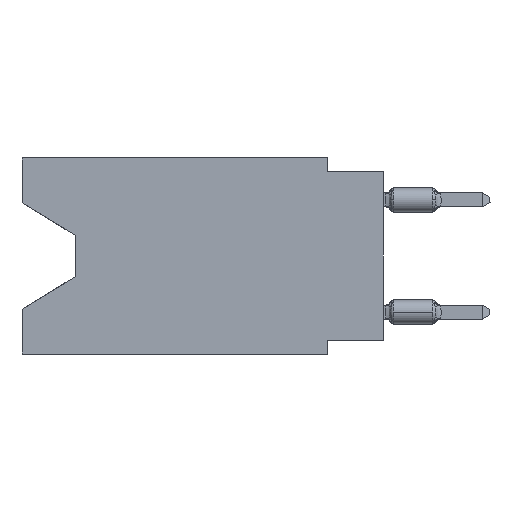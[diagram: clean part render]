
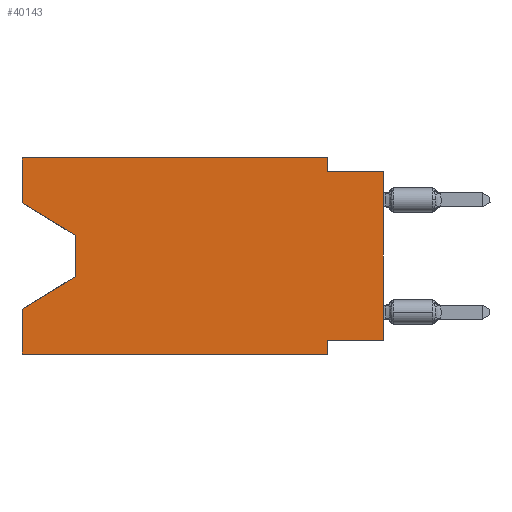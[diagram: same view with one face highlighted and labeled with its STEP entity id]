
A CAD part, left-side view. The second image highlights one B-rep face of the part: STEP entity #40143.
In plain terms, the highlighted planar face has unit normal (-1, 0, 0).
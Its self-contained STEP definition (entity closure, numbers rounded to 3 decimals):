
#113 = LINE ( 'NONE', #17039, #24678 ) ;
#588 = VERTEX_POINT ( 'NONE', #21056 ) ;
#630 = EDGE_CURVE ( 'NONE', #1290, #9018, #39254, .T. ) ;
#1038 = ORIENTED_EDGE ( 'NONE', *, *, #38472, .T. ) ;
#1092 = DIRECTION ( 'NONE',  ( 0., 0., 1. ) ) ;
#1290 = VERTEX_POINT ( 'NONE', #27605 ) ;
#1809 = VECTOR ( 'NONE', #13258, 1000. ) ;
#1930 = ORIENTED_EDGE ( 'NONE', *, *, #27850, .T. ) ;
#2614 = ORIENTED_EDGE ( 'NONE', *, *, #630, .F. ) ;
#5029 = PLANE ( 'NONE',  #36542 ) ;
#5314 = VECTOR ( 'NONE', #26515, 1000. ) ;
#5423 = VERTEX_POINT ( 'NONE', #18499 ) ;
#5823 = LINE ( 'NONE', #12523, #5314 ) ;
#5864 = LINE ( 'NONE', #8759, #38776 ) ;
#7186 = EDGE_CURVE ( 'NONE', #26577, #5423, #24933, .T. ) ;
#7244 = CARTESIAN_POINT ( 'NONE',  ( 0., 16.383, 0. ) ) ;
#7742 = CARTESIAN_POINT ( 'NONE',  ( 0., 0., -8.255 ) ) ;
#8458 = VECTOR ( 'NONE', #39185, 1000. ) ;
#8560 = DIRECTION ( 'NONE',  ( 0., 0., -1. ) ) ;
#8759 = CARTESIAN_POINT ( 'NONE',  ( 0., 13.97, -5.385 ) ) ;
#8957 = EDGE_CURVE ( 'NONE', #38007, #27859, #5823, .T. ) ;
#9018 = VERTEX_POINT ( 'NONE', #19012 ) ;
#9893 = VECTOR ( 'NONE', #8560, 1000. ) ;
#10356 = EDGE_CURVE ( 'NONE', #5423, #12263, #5864, .T. ) ;
#10676 = VERTEX_POINT ( 'NONE', #42977 ) ;
#11389 = LINE ( 'NONE', #31603, #1809 ) ;
#12263 = VERTEX_POINT ( 'NONE', #33851 ) ;
#12523 = CARTESIAN_POINT ( 'NONE',  ( 0., 0., -0.635 ) ) ;
#12874 = CARTESIAN_POINT ( 'NONE',  ( 0., 16.383, 0. ) ) ;
#13258 = DIRECTION ( 'NONE',  ( 0., 0., 1. ) ) ;
#13326 = EDGE_CURVE ( 'NONE', #35288, #12263, #11389, .T. ) ;
#13667 = CARTESIAN_POINT ( 'NONE',  ( 0., 13.97, -3.505 ) ) ;
#14583 = VERTEX_POINT ( 'NONE', #33932 ) ;
#15830 = CARTESIAN_POINT ( 'NONE',  ( 0., 2.54, 0. ) ) ;
#16354 = VERTEX_POINT ( 'NONE', #7742 ) ;
#16783 = VECTOR ( 'NONE', #21916, 1000. ) ;
#17039 = CARTESIAN_POINT ( 'NONE',  ( 0., 16.383, -8.89 ) ) ;
#17949 = ORIENTED_EDGE ( 'NONE', *, *, #13326, .F. ) ;
#18113 = VECTOR ( 'NONE', #25569, 1000. ) ;
#18206 = VECTOR ( 'NONE', #1092, 1000. ) ;
#18499 = CARTESIAN_POINT ( 'NONE',  ( 0., 13.97, -5.385 ) ) ;
#18603 = CARTESIAN_POINT ( 'NONE',  ( 0., 16.383, 0. ) ) ;
#18662 = CARTESIAN_POINT ( 'NONE',  ( 0., 0., 0. ) ) ;
#18694 = CARTESIAN_POINT ( 'NONE',  ( 0., 13.97, -3.505 ) ) ;
#18727 = LINE ( 'NONE', #15830, #8458 ) ;
#18799 = CARTESIAN_POINT ( 'NONE',  ( 0., 2.54, -8.89 ) ) ;
#19012 = CARTESIAN_POINT ( 'NONE',  ( 0., 2.54, -8.89 ) ) ;
#20258 = EDGE_CURVE ( 'NONE', #14583, #588, #43354, .T. ) ;
#20448 = CARTESIAN_POINT ( 'NONE',  ( 0., 0., -0.635 ) ) ;
#20654 = VECTOR ( 'NONE', #26421, 1000. ) ;
#20828 = DIRECTION ( 'NONE',  ( 0., 0., 1. ) ) ;
#21056 = CARTESIAN_POINT ( 'NONE',  ( 0., 2.54, 0. ) ) ;
#21603 = EDGE_CURVE ( 'NONE', #10676, #14583, #27075, .T. ) ;
#21916 = DIRECTION ( 'NONE',  ( 0., -0.855, -0.519 ) ) ;
#21948 = FACE_OUTER_BOUND ( 'NONE', #24569, .T. ) ;
#22223 = LINE ( 'NONE', #42487, #18113 ) ;
#23907 = DIRECTION ( 'NONE',  ( 0., -1., 0. ) ) ;
#23985 = DIRECTION ( 'NONE',  ( 0., 0., -1. ) ) ;
#24569 = EDGE_LOOP ( 'NONE', ( #1930, #37198, #30678, #17949, #1038, #2614, #41704, #26914, #26641, #42467, #36585, #42893 ) ) ;
#24678 = VECTOR ( 'NONE', #23907, 1000. ) ;
#24933 = LINE ( 'NONE', #18694, #37962 ) ;
#25569 = DIRECTION ( 'NONE',  ( 0., 1., 0. ) ) ;
#26421 = DIRECTION ( 'NONE',  ( 0., -1., 0. ) ) ;
#26515 = DIRECTION ( 'NONE',  ( 0., -1., 0. ) ) ;
#26577 = VERTEX_POINT ( 'NONE', #13667 ) ;
#26641 = ORIENTED_EDGE ( 'NONE', *, *, #8957, .F. ) ;
#26914 = ORIENTED_EDGE ( 'NONE', *, *, #28625, .T. ) ;
#27075 = LINE ( 'NONE', #7244, #40613 ) ;
#27605 = CARTESIAN_POINT ( 'NONE',  ( 0., 2.54, -8.255 ) ) ;
#27850 = EDGE_CURVE ( 'NONE', #10676, #26577, #34002, .T. ) ;
#27859 = VERTEX_POINT ( 'NONE', #20448 ) ;
#28585 = CARTESIAN_POINT ( 'NONE',  ( 0., 2.54, -0.635 ) ) ;
#28625 = EDGE_CURVE ( 'NONE', #16354, #27859, #28896, .T. ) ;
#28896 = LINE ( 'NONE', #18662, #18206 ) ;
#29688 = DIRECTION ( 'NONE',  ( 0., 0.855, -0.519 ) ) ;
#30678 = ORIENTED_EDGE ( 'NONE', *, *, #10356, .T. ) ;
#31603 = CARTESIAN_POINT ( 'NONE',  ( 0., 16.383, 0. ) ) ;
#32148 = DIRECTION ( 'NONE',  ( 1., 0., 0. ) ) ;
#33851 = CARTESIAN_POINT ( 'NONE',  ( 0., 16.383, -6.852 ) ) ;
#33932 = CARTESIAN_POINT ( 'NONE',  ( 0., 16.383, 0. ) ) ;
#34002 = LINE ( 'NONE', #42380, #16783 ) ;
#34415 = EDGE_CURVE ( 'NONE', #588, #38007, #18727, .T. ) ;
#34551 = CARTESIAN_POINT ( 'NONE',  ( 0., 16.383, -8.89 ) ) ;
#35288 = VERTEX_POINT ( 'NONE', #34551 ) ;
#36542 = AXIS2_PLACEMENT_3D ( 'NONE', #18603, #32148, #23985 ) ;
#36585 = ORIENTED_EDGE ( 'NONE', *, *, #20258, .F. ) ;
#37198 = ORIENTED_EDGE ( 'NONE', *, *, #7186, .T. ) ;
#37962 = VECTOR ( 'NONE', #42510, 1000. ) ;
#38007 = VERTEX_POINT ( 'NONE', #28585 ) ;
#38472 = EDGE_CURVE ( 'NONE', #35288, #9018, #113, .T. ) ;
#38776 = VECTOR ( 'NONE', #29688, 1000. ) ;
#39185 = DIRECTION ( 'NONE',  ( 0., 0., -1. ) ) ;
#39254 = LINE ( 'NONE', #18799, #9893 ) ;
#40143 = ADVANCED_FACE ( 'NONE', ( #21948 ), #5029, .F. ) ;
#40613 = VECTOR ( 'NONE', #20828, 1000. ) ;
#41704 = ORIENTED_EDGE ( 'NONE', *, *, #42107, .F. ) ;
#42107 = EDGE_CURVE ( 'NONE', #16354, #1290, #22223, .T. ) ;
#42380 = CARTESIAN_POINT ( 'NONE',  ( 0., 16.383, -2.038 ) ) ;
#42467 = ORIENTED_EDGE ( 'NONE', *, *, #34415, .F. ) ;
#42487 = CARTESIAN_POINT ( 'NONE',  ( 0., 0., -8.255 ) ) ;
#42510 = DIRECTION ( 'NONE',  ( 0., 0., -1. ) ) ;
#42893 = ORIENTED_EDGE ( 'NONE', *, *, #21603, .F. ) ;
#42977 = CARTESIAN_POINT ( 'NONE',  ( 0., 16.383, -2.038 ) ) ;
#43354 = LINE ( 'NONE', #12874, #20654 ) ;
